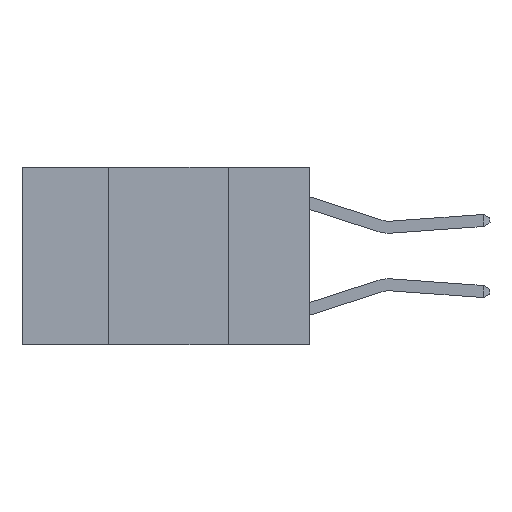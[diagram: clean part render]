
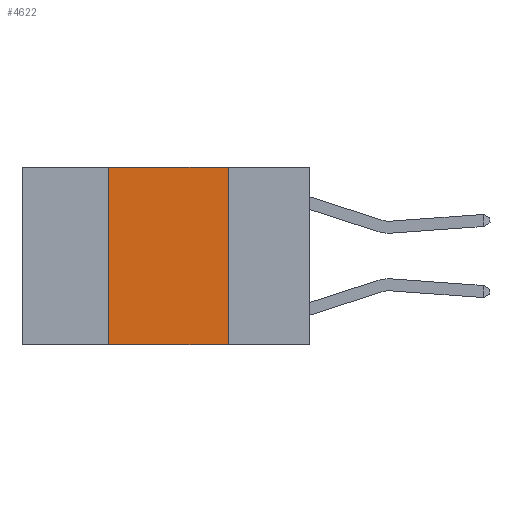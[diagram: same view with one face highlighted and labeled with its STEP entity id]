
A CAD part, left-side view. The second image highlights one B-rep face of the part: STEP entity #4622.
In plain terms, the highlighted planar face has unit normal (-1, 0, 0).
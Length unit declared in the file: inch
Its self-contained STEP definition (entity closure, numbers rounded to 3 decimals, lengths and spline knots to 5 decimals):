
#21 = VECTOR ( 'NONE', #9520, 39.37008 ) ;
#257 = VECTOR ( 'NONE', #5353, 39.37008 ) ;
#404 = CARTESIAN_POINT ( 'NONE',  ( 0., 0.6, 0. ) ) ;
#474 = DIRECTION ( 'NONE',  ( 0., 0., -1. ) ) ;
#791 = ORIENTED_EDGE ( 'NONE', *, *, #11320, .F. ) ;
#2387 = CARTESIAN_POINT ( 'NONE',  ( 0., 0.17, -0.37 ) ) ;
#2460 = CARTESIAN_POINT ( 'NONE',  ( 0., 0.42, 0. ) ) ;
#3946 = VECTOR ( 'NONE', #4496, 39.37008 ) ;
#4496 = DIRECTION ( 'NONE',  ( 0., 0., -1. ) ) ;
#4598 = LINE ( 'NONE', #2460, #257 ) ;
#4622 = ADVANCED_FACE ( 'NONE', ( #16590 ), #18222, .F. ) ;
#5353 = DIRECTION ( 'NONE',  ( 0., 0., 1. ) ) ;
#7258 = LINE ( 'NONE', #14199, #3946 ) ;
#8598 = EDGE_CURVE ( 'NONE', #20529, #11331, #7258, .T. ) ;
#9248 = VECTOR ( 'NONE', #12127, 39.37008 ) ;
#9520 = DIRECTION ( 'NONE',  ( 0., -1., 0. ) ) ;
#9565 = ORIENTED_EDGE ( 'NONE', *, *, #20796, .F. ) ;
#10316 = DIRECTION ( 'NONE',  ( 1., 0., 0. ) ) ;
#10332 = CARTESIAN_POINT ( 'NONE',  ( 0., 0.42, -0.37 ) ) ;
#10914 = EDGE_CURVE ( 'NONE', #18050, #11331, #11517, .T. ) ;
#11320 = EDGE_CURVE ( 'NONE', #15471, #20529, #16716, .T. ) ;
#11322 = CARTESIAN_POINT ( 'NONE',  ( 0., 0.17, 0. ) ) ;
#11331 = VERTEX_POINT ( 'NONE', #2387 ) ;
#11517 = LINE ( 'NONE', #12715, #21 ) ;
#11585 = AXIS2_PLACEMENT_3D ( 'NONE', #404, #10316, #474 ) ;
#12061 = CARTESIAN_POINT ( 'NONE',  ( 0., 0.6, 0. ) ) ;
#12127 = DIRECTION ( 'NONE',  ( 0., -1., 0. ) ) ;
#12715 = CARTESIAN_POINT ( 'NONE',  ( 0., 0.6, -0.37 ) ) ;
#13285 = ORIENTED_EDGE ( 'NONE', *, *, #8598, .F. ) ;
#14199 = CARTESIAN_POINT ( 'NONE',  ( 0., 0.17, 0. ) ) ;
#14750 = CARTESIAN_POINT ( 'NONE',  ( 0., 0.42, 0. ) ) ;
#14968 = EDGE_LOOP ( 'NONE', ( #13285, #791, #9565, #18013 ) ) ;
#15471 = VERTEX_POINT ( 'NONE', #14750 ) ;
#16590 = FACE_OUTER_BOUND ( 'NONE', #14968, .T. ) ;
#16716 = LINE ( 'NONE', #12061, #9248 ) ;
#18013 = ORIENTED_EDGE ( 'NONE', *, *, #10914, .T. ) ;
#18050 = VERTEX_POINT ( 'NONE', #10332 ) ;
#18222 = PLANE ( 'NONE',  #11585 ) ;
#20529 = VERTEX_POINT ( 'NONE', #11322 ) ;
#20796 = EDGE_CURVE ( 'NONE', #18050, #15471, #4598, .T. ) ;
